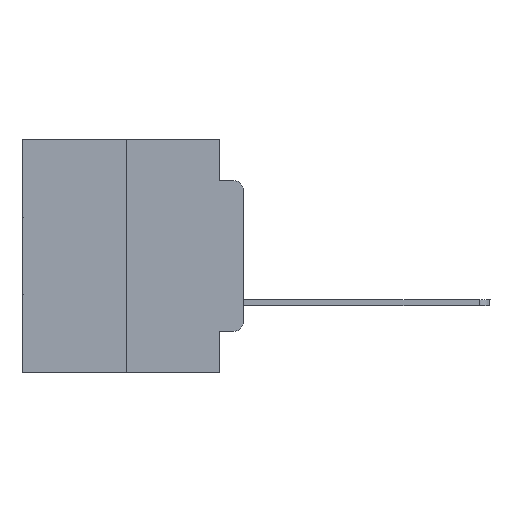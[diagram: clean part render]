
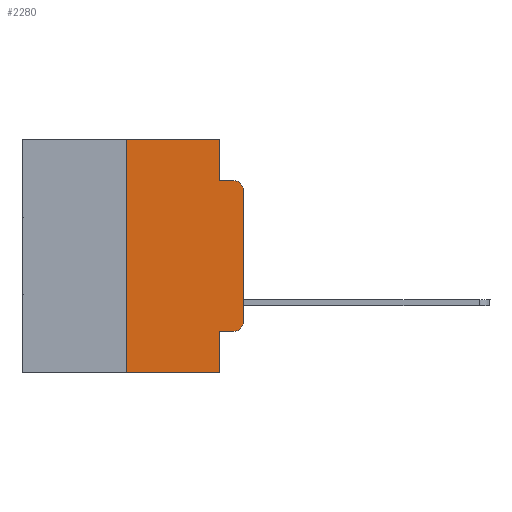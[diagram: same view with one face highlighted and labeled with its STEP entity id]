
A CAD part, left-side view. The second image highlights one B-rep face of the part: STEP entity #2280.
In plain terms, the highlighted planar face has unit normal (-1, 0, 0).
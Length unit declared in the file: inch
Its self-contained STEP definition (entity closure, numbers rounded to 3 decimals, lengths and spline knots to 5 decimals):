
#65 = CARTESIAN_POINT ( 'NONE',  ( 0., 0.473, 0. ) ) ;
#243 = AXIS2_PLACEMENT_3D ( 'NONE', #8199, #17131, #21165 ) ;
#375 = CARTESIAN_POINT ( 'NONE',  ( 0., 0.25, 0. ) ) ;
#816 = EDGE_CURVE ( 'NONE', #18807, #6453, #6113, .T. ) ;
#971 = AXIS2_PLACEMENT_3D ( 'NONE', #65, #2318, #15021 ) ;
#1233 = CARTESIAN_POINT ( 'NONE',  ( 0., 0.25, -0.5 ) ) ;
#1282 = VECTOR ( 'NONE', #18437, 39.37008 ) ;
#1451 = ORIENTED_EDGE ( 'NONE', *, *, #14765, .F. ) ;
#1633 = CARTESIAN_POINT ( 'NONE',  ( 0., 0.051, 0. ) ) ;
#2280 = ADVANCED_FACE ( 'NONE', ( #10089 ), #12860, .F. ) ;
#2318 = DIRECTION ( 'NONE',  ( 1., 0., 0. ) ) ;
#3046 = CARTESIAN_POINT ( 'NONE',  ( 0., 0., 0. ) ) ;
#3121 = EDGE_CURVE ( 'NONE', #8262, #25366, #15713, .T. ) ;
#3242 = LINE ( 'NONE', #13484, #25512 ) ;
#3310 = LINE ( 'NONE', #27084, #1282 ) ;
#3527 = AXIS2_PLACEMENT_3D ( 'NONE', #17097, #23469, #25694 ) ;
#3910 = ORIENTED_EDGE ( 'NONE', *, *, #11486, .F. ) ;
#3976 = LINE ( 'NONE', #3046, #21212 ) ;
#4319 = CARTESIAN_POINT ( 'NONE',  ( 0., 0.473, -0.5 ) ) ;
#4382 = EDGE_CURVE ( 'NONE', #22839, #7982, #15665, .T. ) ;
#5041 = CARTESIAN_POINT ( 'NONE',  ( 0., 0.051, -0.5 ) ) ;
#5057 = ORIENTED_EDGE ( 'NONE', *, *, #3121, .F. ) ;
#5490 = CARTESIAN_POINT ( 'NONE',  ( 0., 0.02, -0.0885 ) ) ;
#5659 = ORIENTED_EDGE ( 'NONE', *, *, #20105, .F. ) ;
#6113 = LINE ( 'NONE', #4319, #22702 ) ;
#6366 = DIRECTION ( 'NONE',  ( 0., 0., -1. ) ) ;
#6453 = VERTEX_POINT ( 'NONE', #5041 ) ;
#6778 = DIRECTION ( 'NONE',  ( 0., -1., 0. ) ) ;
#6796 = ORIENTED_EDGE ( 'NONE', *, *, #24471, .T. ) ;
#7982 = VERTEX_POINT ( 'NONE', #18584 ) ;
#8191 = EDGE_CURVE ( 'NONE', #7982, #18802, #3976, .T. ) ;
#8199 = CARTESIAN_POINT ( 'NONE',  ( 0., 0.02, -0.1085 ) ) ;
#8262 = VERTEX_POINT ( 'NONE', #1633 ) ;
#8635 = DIRECTION ( 'NONE',  ( 0., -1., 0. ) ) ;
#9977 = VECTOR ( 'NONE', #18189, 39.37008 ) ;
#10089 = FACE_OUTER_BOUND ( 'NONE', #23989, .T. ) ;
#10512 = VECTOR ( 'NONE', #13491, 39.37008 ) ;
#10749 = CARTESIAN_POINT ( 'NONE',  ( 0., 0.051, -0.0885 ) ) ;
#11170 = CARTESIAN_POINT ( 'NONE',  ( 0., 0.051, -0.4115 ) ) ;
#11486 = EDGE_CURVE ( 'NONE', #18807, #18406, #17894, .T. ) ;
#12170 = VECTOR ( 'NONE', #19809, 39.37008 ) ;
#12469 = ORIENTED_EDGE ( 'NONE', *, *, #21472, .F. ) ;
#12860 = PLANE ( 'NONE',  #971 ) ;
#13484 = CARTESIAN_POINT ( 'NONE',  ( 0., 0.051, -0.0885 ) ) ;
#13491 = DIRECTION ( 'NONE',  ( 0., -1., 0. ) ) ;
#13518 = VERTEX_POINT ( 'NONE', #5490 ) ;
#13923 = EDGE_CURVE ( 'NONE', #18802, #13518, #21530, .T. ) ;
#14480 = CARTESIAN_POINT ( 'NONE',  ( 0., 0., -0.1085 ) ) ;
#14765 = EDGE_CURVE ( 'NONE', #25366, #13518, #3242, .T. ) ;
#14863 = LINE ( 'NONE', #19839, #10512 ) ;
#15021 = DIRECTION ( 'NONE',  ( 0., 0., -1. ) ) ;
#15665 = CIRCLE ( 'NONE', #3527, 0.02 ) ;
#15713 = LINE ( 'NONE', #24786, #9977 ) ;
#15769 = VECTOR ( 'NONE', #6366, 39.37008 ) ;
#15778 = ORIENTED_EDGE ( 'NONE', *, *, #13923, .T. ) ;
#17097 = CARTESIAN_POINT ( 'NONE',  ( 0., 0.02, -0.3915 ) ) ;
#17131 = DIRECTION ( 'NONE',  ( -1., 0., 0. ) ) ;
#17894 = LINE ( 'NONE', #375, #12170 ) ;
#18136 = DIRECTION ( 'NONE',  ( 0., 0., 1. ) ) ;
#18189 = DIRECTION ( 'NONE',  ( 0., 0., -1. ) ) ;
#18406 = VERTEX_POINT ( 'NONE', #18606 ) ;
#18437 = DIRECTION ( 'NONE',  ( 0., -1., 0. ) ) ;
#18584 = CARTESIAN_POINT ( 'NONE',  ( 0., 0., -0.3915 ) ) ;
#18606 = CARTESIAN_POINT ( 'NONE',  ( 0., 0.25, 0. ) ) ;
#18802 = VERTEX_POINT ( 'NONE', #14480 ) ;
#18807 = VERTEX_POINT ( 'NONE', #1233 ) ;
#19275 = ORIENTED_EDGE ( 'NONE', *, *, #4382, .T. ) ;
#19809 = DIRECTION ( 'NONE',  ( 0., 0., 1. ) ) ;
#19839 = CARTESIAN_POINT ( 'NONE',  ( 0., 0.473, 0. ) ) ;
#20105 = EDGE_CURVE ( 'NONE', #26226, #6453, #20189, .T. ) ;
#20182 = ORIENTED_EDGE ( 'NONE', *, *, #8191, .T. ) ;
#20189 = LINE ( 'NONE', #26156, #15769 ) ;
#20720 = ORIENTED_EDGE ( 'NONE', *, *, #816, .T. ) ;
#21165 = DIRECTION ( 'NONE',  ( 0., 0., -1. ) ) ;
#21212 = VECTOR ( 'NONE', #18136, 39.37008 ) ;
#21472 = EDGE_CURVE ( 'NONE', #18406, #8262, #14863, .T. ) ;
#21530 = CIRCLE ( 'NONE', #243, 0.02 ) ;
#22702 = VECTOR ( 'NONE', #8635, 39.37008 ) ;
#22839 = VERTEX_POINT ( 'NONE', #23628 ) ;
#23469 = DIRECTION ( 'NONE',  ( -1., 0., 0. ) ) ;
#23628 = CARTESIAN_POINT ( 'NONE',  ( 0., 0.02, -0.4115 ) ) ;
#23989 = EDGE_LOOP ( 'NONE', ( #20182, #15778, #1451, #5057, #12469, #3910, #20720, #5659, #6796, #19275 ) ) ;
#24471 = EDGE_CURVE ( 'NONE', #26226, #22839, #3310, .T. ) ;
#24786 = CARTESIAN_POINT ( 'NONE',  ( 0., 0.051, 0. ) ) ;
#25366 = VERTEX_POINT ( 'NONE', #10749 ) ;
#25512 = VECTOR ( 'NONE', #6778, 39.37008 ) ;
#25694 = DIRECTION ( 'NONE',  ( 0., 0., -1. ) ) ;
#26156 = CARTESIAN_POINT ( 'NONE',  ( 0., 0.051, 0. ) ) ;
#26226 = VERTEX_POINT ( 'NONE', #11170 ) ;
#27084 = CARTESIAN_POINT ( 'NONE',  ( 0., 0.051, -0.4115 ) ) ;
